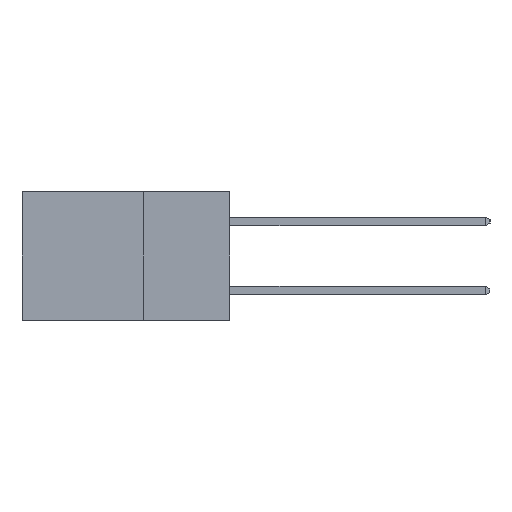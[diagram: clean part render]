
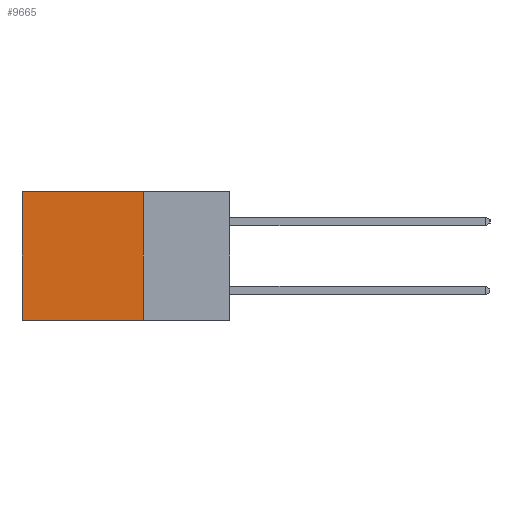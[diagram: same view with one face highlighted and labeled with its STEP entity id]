
A CAD part, left-side view. The second image highlights one B-rep face of the part: STEP entity #9665.
In plain terms, the highlighted planar face has unit normal (-1, 0, 0).
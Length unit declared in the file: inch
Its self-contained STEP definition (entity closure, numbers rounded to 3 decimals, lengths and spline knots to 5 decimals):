
#183 = PLANE ( 'NONE',  #7962 ) ;
#751 = VERTEX_POINT ( 'NONE', #3033 ) ;
#872 = VECTOR ( 'NONE', #12478, 39.37008 ) ;
#1470 = EDGE_CURVE ( 'NONE', #11594, #4366, #9827, .T. ) ;
#1500 = EDGE_CURVE ( 'NONE', #4366, #10702, #1541, .T. ) ;
#1541 = LINE ( 'NONE', #12175, #6415 ) ;
#2347 = CARTESIAN_POINT ( 'NONE',  ( 0.298, 0.25, 0. ) ) ;
#2364 = CARTESIAN_POINT ( 'NONE',  ( 0.298, 0.25, -0.37 ) ) ;
#3033 = CARTESIAN_POINT ( 'NONE',  ( 0.298, 0.6, 0. ) ) ;
#3746 = VECTOR ( 'NONE', #10911, 39.37008 ) ;
#4313 = VECTOR ( 'NONE', #11235, 39.37008 ) ;
#4366 = VERTEX_POINT ( 'NONE', #2364 ) ;
#4449 = ORIENTED_EDGE ( 'NONE', *, *, #1500, .F. ) ;
#4673 = EDGE_LOOP ( 'NONE', ( #4839, #4449, #4799, #11668 ) ) ;
#4799 = ORIENTED_EDGE ( 'NONE', *, *, #1470, .F. ) ;
#4839 = ORIENTED_EDGE ( 'NONE', *, *, #5099, .T. ) ;
#5099 = EDGE_CURVE ( 'NONE', #751, #10702, #9248, .T. ) ;
#5198 = CARTESIAN_POINT ( 'NONE',  ( 0.298, 0.25, 0. ) ) ;
#5489 = DIRECTION ( 'NONE',  ( 1., 0., 0. ) ) ;
#5854 = CARTESIAN_POINT ( 'NONE',  ( 0.298, 0.6, -0.37 ) ) ;
#6415 = VECTOR ( 'NONE', #9396, 39.37008 ) ;
#6502 = CARTESIAN_POINT ( 'NONE',  ( 0.298, 0.25, 0. ) ) ;
#7790 = CARTESIAN_POINT ( 'NONE',  ( 0.298, 0.6, 0. ) ) ;
#7962 = AXIS2_PLACEMENT_3D ( 'NONE', #2347, #5489, #12780 ) ;
#7967 = CARTESIAN_POINT ( 'NONE',  ( 0.298, 0.25, 0. ) ) ;
#9248 = LINE ( 'NONE', #7790, #3746 ) ;
#9396 = DIRECTION ( 'NONE',  ( 0., 1., 0. ) ) ;
#9665 = ADVANCED_FACE ( 'NONE', ( #11660 ), #183, .F. ) ;
#9827 = LINE ( 'NONE', #7967, #4313 ) ;
#10126 = EDGE_CURVE ( 'NONE', #11594, #751, #11649, .T. ) ;
#10702 = VERTEX_POINT ( 'NONE', #5854 ) ;
#10911 = DIRECTION ( 'NONE',  ( 0., 0., -1. ) ) ;
#11235 = DIRECTION ( 'NONE',  ( 0., 0., -1. ) ) ;
#11594 = VERTEX_POINT ( 'NONE', #6502 ) ;
#11649 = LINE ( 'NONE', #5198, #872 ) ;
#11660 = FACE_OUTER_BOUND ( 'NONE', #4673, .T. ) ;
#11668 = ORIENTED_EDGE ( 'NONE', *, *, #10126, .T. ) ;
#12175 = CARTESIAN_POINT ( 'NONE',  ( 0.298, 0.25, -0.37 ) ) ;
#12478 = DIRECTION ( 'NONE',  ( 0., 1., 0. ) ) ;
#12780 = DIRECTION ( 'NONE',  ( 0., 0., -1. ) ) ;
